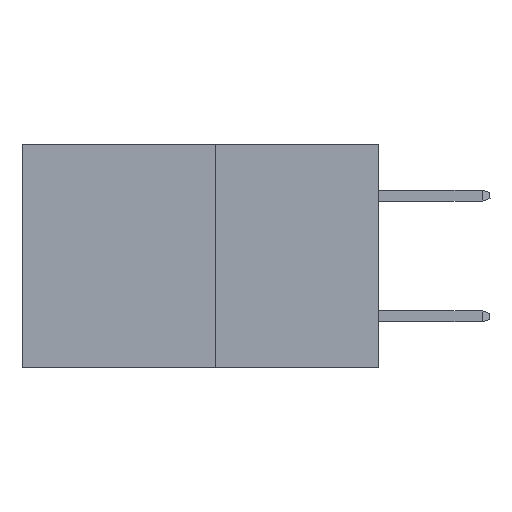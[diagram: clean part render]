
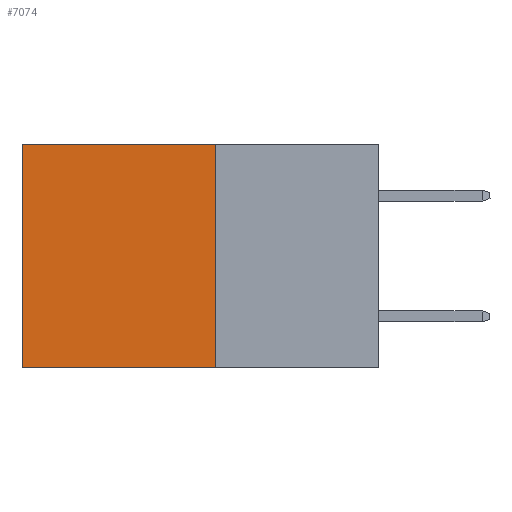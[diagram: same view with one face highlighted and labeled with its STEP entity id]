
A CAD part, left-side view. The second image highlights one B-rep face of the part: STEP entity #7074.
In plain terms, the highlighted planar face has unit normal (-1, 0, 0).
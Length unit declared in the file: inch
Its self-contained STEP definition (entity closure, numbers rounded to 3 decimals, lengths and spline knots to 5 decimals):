
#11 = DIRECTION ( 'NONE',  ( 0., 1., 0. ) ) ;
#41 = VERTEX_POINT ( 'NONE', #6629 ) ;
#191 = DIRECTION ( 'NONE',  ( 1., 0., 0. ) ) ;
#203 = CARTESIAN_POINT ( 'NONE',  ( 0.277, 0.27, -0.37 ) ) ;
#717 = DIRECTION ( 'NONE',  ( 0., 0., -1. ) ) ;
#876 = AXIS2_PLACEMENT_3D ( 'NONE', #203, #191, #3629 ) ;
#1501 = CARTESIAN_POINT ( 'NONE',  ( 0.277, 0.27, -0.37 ) ) ;
#1605 = VECTOR ( 'NONE', #11, 39.37008 ) ;
#1719 = VERTEX_POINT ( 'NONE', #1501 ) ;
#1861 = CARTESIAN_POINT ( 'NONE',  ( 0.277, 0.59, -0.37 ) ) ;
#1909 = ORIENTED_EDGE ( 'NONE', *, *, #2209, .F. ) ;
#2209 = EDGE_CURVE ( 'NONE', #1719, #6407, #2550, .T. ) ;
#2280 = LINE ( 'NONE', #7489, #6631 ) ;
#2550 = LINE ( 'NONE', #6400, #6992 ) ;
#2991 = ORIENTED_EDGE ( 'NONE', *, *, #7528, .T. ) ;
#3439 = LINE ( 'NONE', #4466, #7729 ) ;
#3582 = ORIENTED_EDGE ( 'NONE', *, *, #5588, .T. ) ;
#3629 = DIRECTION ( 'NONE',  ( 0., 0., -1. ) ) ;
#3908 = FACE_OUTER_BOUND ( 'NONE', #4227, .T. ) ;
#4227 = EDGE_LOOP ( 'NONE', ( #3582, #1909, #4234, #2991 ) ) ;
#4234 = ORIENTED_EDGE ( 'NONE', *, *, #6163, .F. ) ;
#4466 = CARTESIAN_POINT ( 'NONE',  ( 0.277, 0.59, -0.37 ) ) ;
#4777 = CARTESIAN_POINT ( 'NONE',  ( 0.277, 0.59, 0. ) ) ;
#5396 = VERTEX_POINT ( 'NONE', #4777 ) ;
#5588 = EDGE_CURVE ( 'NONE', #5396, #6407, #3439, .T. ) ;
#5928 = LINE ( 'NONE', #7301, #1605 ) ;
#6163 = EDGE_CURVE ( 'NONE', #41, #1719, #2280, .T. ) ;
#6400 = CARTESIAN_POINT ( 'NONE',  ( 0.277, 0.27, -0.37 ) ) ;
#6407 = VERTEX_POINT ( 'NONE', #1861 ) ;
#6534 = DIRECTION ( 'NONE',  ( 0., 0., -1. ) ) ;
#6629 = CARTESIAN_POINT ( 'NONE',  ( 0.277, 0.27, 0. ) ) ;
#6631 = VECTOR ( 'NONE', #6534, 39.37008 ) ;
#6946 = PLANE ( 'NONE',  #876 ) ;
#6992 = VECTOR ( 'NONE', #7053, 39.37008 ) ;
#7053 = DIRECTION ( 'NONE',  ( 0., 1., 0. ) ) ;
#7074 = ADVANCED_FACE ( 'NONE', ( #3908 ), #6946, .F. ) ;
#7301 = CARTESIAN_POINT ( 'NONE',  ( 0.277, 0.27, 0. ) ) ;
#7489 = CARTESIAN_POINT ( 'NONE',  ( 0.277, 0.27, -0.37 ) ) ;
#7528 = EDGE_CURVE ( 'NONE', #41, #5396, #5928, .T. ) ;
#7729 = VECTOR ( 'NONE', #717, 39.37008 ) ;
